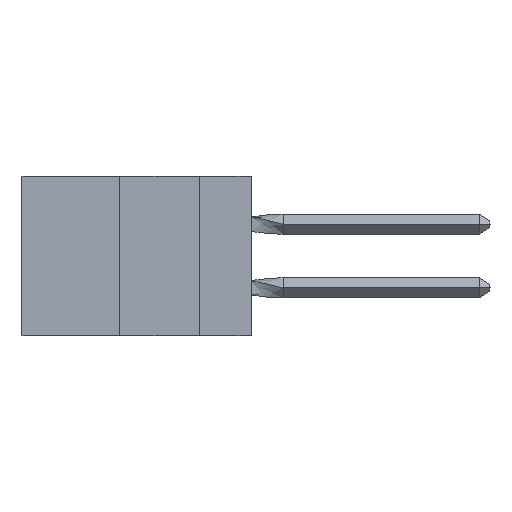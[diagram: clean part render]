
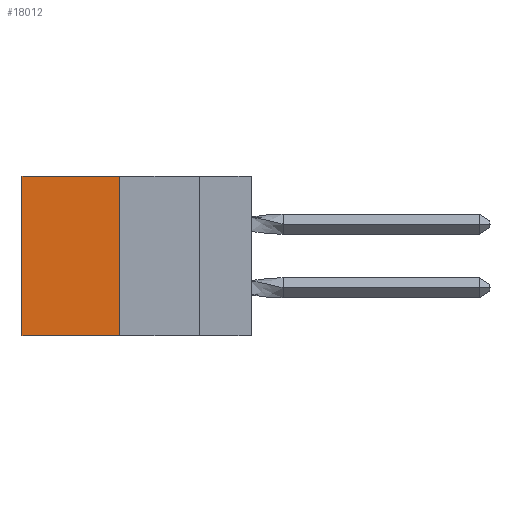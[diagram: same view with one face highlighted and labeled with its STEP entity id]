
A CAD part, left-side view. The second image highlights one B-rep face of the part: STEP entity #18012.
In plain terms, the highlighted planar face has unit normal (-1, 0, 0).
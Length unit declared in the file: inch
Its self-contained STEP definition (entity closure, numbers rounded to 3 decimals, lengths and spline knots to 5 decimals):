
#293 = CARTESIAN_POINT ( 'NONE',  ( 0.305, 0.413, -0.5 ) ) ;
#1719 = DIRECTION ( 'NONE',  ( 0., 0., -1. ) ) ;
#2152 = VECTOR ( 'NONE', #25765, 39.37008 ) ;
#3956 = ORIENTED_EDGE ( 'NONE', *, *, #30272, .F. ) ;
#6677 = CARTESIAN_POINT ( 'NONE',  ( 0.305, 0.413, -0.5 ) ) ;
#6691 = DIRECTION ( 'NONE',  ( 0., 0., -1. ) ) ;
#6955 = VECTOR ( 'NONE', #29633, 39.37008 ) ;
#7653 = ORIENTED_EDGE ( 'NONE', *, *, #34131, .T. ) ;
#7844 = CARTESIAN_POINT ( 'NONE',  ( 0.305, 0.72, -0.5 ) ) ;
#8793 = LINE ( 'NONE', #7844, #30701 ) ;
#10126 = AXIS2_PLACEMENT_3D ( 'NONE', #293, #32334, #6691 ) ;
#10203 = VERTEX_POINT ( 'NONE', #29310 ) ;
#12919 = CARTESIAN_POINT ( 'NONE',  ( 0.305, 0.413, -0.5 ) ) ;
#13567 = LINE ( 'NONE', #12919, #2152 ) ;
#15875 = EDGE_CURVE ( 'NONE', #22840, #20789, #8793, .T. ) ;
#15996 = VERTEX_POINT ( 'NONE', #6677 ) ;
#18012 = ADVANCED_FACE ( 'NONE', ( #31818 ), #35251, .F. ) ;
#20457 = DIRECTION ( 'NONE',  ( 0., 1., 0. ) ) ;
#20789 = VERTEX_POINT ( 'NONE', #23121 ) ;
#21539 = EDGE_CURVE ( 'NONE', #10203, #15996, #13567, .T. ) ;
#22840 = VERTEX_POINT ( 'NONE', #25576 ) ;
#23121 = CARTESIAN_POINT ( 'NONE',  ( 0.305, 0.72, -0.5 ) ) ;
#23938 = LINE ( 'NONE', #27543, #6955 ) ;
#25324 = VECTOR ( 'NONE', #20457, 39.37008 ) ;
#25576 = CARTESIAN_POINT ( 'NONE',  ( 0.305, 0.72, 0. ) ) ;
#25765 = DIRECTION ( 'NONE',  ( 0., 0., -1. ) ) ;
#27543 = CARTESIAN_POINT ( 'NONE',  ( 0.305, 0.413, 0. ) ) ;
#28690 = ORIENTED_EDGE ( 'NONE', *, *, #21539, .F. ) ;
#28753 = EDGE_LOOP ( 'NONE', ( #31786, #3956, #28690, #7653 ) ) ;
#29310 = CARTESIAN_POINT ( 'NONE',  ( 0.305, 0.413, 0. ) ) ;
#29633 = DIRECTION ( 'NONE',  ( 0., 1., 0. ) ) ;
#30272 = EDGE_CURVE ( 'NONE', #15996, #20789, #35813, .T. ) ;
#30701 = VECTOR ( 'NONE', #1719, 39.37008 ) ;
#31786 = ORIENTED_EDGE ( 'NONE', *, *, #15875, .T. ) ;
#31818 = FACE_OUTER_BOUND ( 'NONE', #28753, .T. ) ;
#32334 = DIRECTION ( 'NONE',  ( 1., 0., 0. ) ) ;
#34131 = EDGE_CURVE ( 'NONE', #10203, #22840, #23938, .T. ) ;
#35251 = PLANE ( 'NONE',  #10126 ) ;
#35813 = LINE ( 'NONE', #36343, #25324 ) ;
#36343 = CARTESIAN_POINT ( 'NONE',  ( 0.305, 0.413, -0.5 ) ) ;
